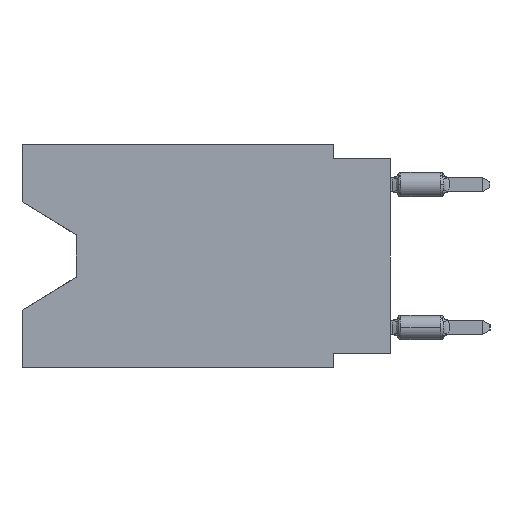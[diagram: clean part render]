
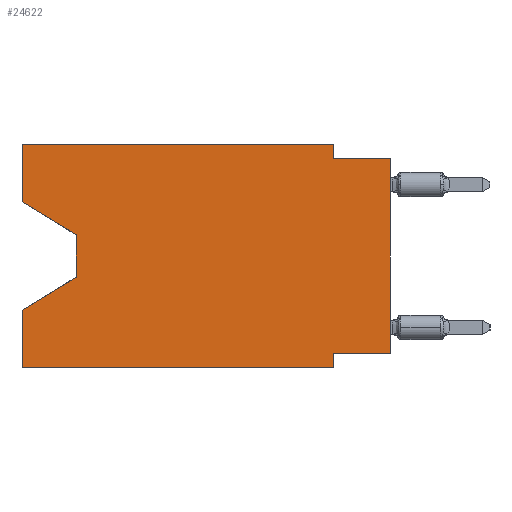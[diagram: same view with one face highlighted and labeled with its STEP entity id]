
A CAD part, left-side view. The second image highlights one B-rep face of the part: STEP entity #24622.
In plain terms, the highlighted planar face has unit normal (-1, 0, 0).
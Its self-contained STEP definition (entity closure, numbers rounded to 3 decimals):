
#47 = LINE ( 'NONE', #8810, #2737 ) ;
#103 = ORIENTED_EDGE ( 'NONE', *, *, #1691, .T. ) ;
#515 = ORIENTED_EDGE ( 'NONE', *, *, #9716, .T. ) ;
#597 = DIRECTION ( 'NONE',  ( 0., -1., 0. ) ) ;
#828 = VECTOR ( 'NONE', #20062, 1000. ) ;
#946 = VECTOR ( 'NONE', #24637, 1000. ) ;
#955 = VECTOR ( 'NONE', #1901, 1000. ) ;
#1691 = EDGE_CURVE ( 'NONE', #12206, #12368, #4442, .T. ) ;
#1764 = DIRECTION ( 'NONE',  ( 0., -1., 0. ) ) ;
#1812 = ORIENTED_EDGE ( 'NONE', *, *, #13598, .F. ) ;
#1901 = DIRECTION ( 'NONE',  ( 0., 0., 1. ) ) ;
#2100 = DIRECTION ( 'NONE',  ( 0., 0., -1. ) ) ;
#2536 = CARTESIAN_POINT ( 'NONE',  ( 0., 13.97, -4.013 ) ) ;
#2659 = CARTESIAN_POINT ( 'NONE',  ( 0., 0., -0.635 ) ) ;
#2737 = VECTOR ( 'NONE', #17561, 1000. ) ;
#2953 = DIRECTION ( 'NONE',  ( 0., 0., 1. ) ) ;
#3055 = VECTOR ( 'NONE', #597, 1000. ) ;
#3444 = VERTEX_POINT ( 'NONE', #13907 ) ;
#3875 = DIRECTION ( 'NONE',  ( 0., -1., 0. ) ) ;
#4442 = LINE ( 'NONE', #6744, #22879 ) ;
#4982 = ORIENTED_EDGE ( 'NONE', *, *, #12960, .F. ) ;
#4999 = CARTESIAN_POINT ( 'NONE',  ( 0., 2.54, -9.906 ) ) ;
#5498 = VERTEX_POINT ( 'NONE', #5629 ) ;
#5627 = CARTESIAN_POINT ( 'NONE',  ( 0., 2.54, -9.906 ) ) ;
#5629 = CARTESIAN_POINT ( 'NONE',  ( 0., 16.383, -7.36 ) ) ;
#5765 = EDGE_CURVE ( 'NONE', #12368, #5498, #17617, .T. ) ;
#6308 = VECTOR ( 'NONE', #7098, 1000. ) ;
#6665 = LINE ( 'NONE', #26929, #946 ) ;
#6677 = CARTESIAN_POINT ( 'NONE',  ( 0., 0., -9.271 ) ) ;
#6744 = CARTESIAN_POINT ( 'NONE',  ( 0., 13.97, -4.013 ) ) ;
#7058 = CARTESIAN_POINT ( 'NONE',  ( 0., 16.383, -9.906 ) ) ;
#7090 = AXIS2_PLACEMENT_3D ( 'NONE', #14928, #23681, #10766 ) ;
#7098 = DIRECTION ( 'NONE',  ( 0., 1., 0. ) ) ;
#7792 = LINE ( 'NONE', #5627, #11280 ) ;
#8624 = EDGE_CURVE ( 'NONE', #17166, #3444, #6665, .T. ) ;
#8719 = CARTESIAN_POINT ( 'NONE',  ( 0., 13.97, -5.893 ) ) ;
#8810 = CARTESIAN_POINT ( 'NONE',  ( 0., 16.383, -2.546 ) ) ;
#9716 = EDGE_CURVE ( 'NONE', #23384, #27047, #22628, .T. ) ;
#9970 = VERTEX_POINT ( 'NONE', #25915 ) ;
#10042 = VERTEX_POINT ( 'NONE', #20410 ) ;
#10766 = DIRECTION ( 'NONE',  ( 0., 0., -1. ) ) ;
#11064 = VECTOR ( 'NONE', #2100, 1000. ) ;
#11280 = VECTOR ( 'NONE', #14399, 1000. ) ;
#11384 = CARTESIAN_POINT ( 'NONE',  ( 0., 16.383, -2.546 ) ) ;
#11503 = VERTEX_POINT ( 'NONE', #23024 ) ;
#11617 = EDGE_CURVE ( 'NONE', #10042, #5498, #12825, .T. ) ;
#12206 = VERTEX_POINT ( 'NONE', #2536 ) ;
#12368 = VERTEX_POINT ( 'NONE', #27376 ) ;
#12781 = PLANE ( 'NONE',  #7090 ) ;
#12825 = LINE ( 'NONE', #25882, #955 ) ;
#12960 = EDGE_CURVE ( 'NONE', #3444, #11503, #19133, .T. ) ;
#13528 = ORIENTED_EDGE ( 'NONE', *, *, #17537, .T. ) ;
#13598 = EDGE_CURVE ( 'NONE', #11503, #18250, #17049, .T. ) ;
#13907 = CARTESIAN_POINT ( 'NONE',  ( 0., 16.383, 0. ) ) ;
#14399 = DIRECTION ( 'NONE',  ( 0., 0., -1. ) ) ;
#14800 = LINE ( 'NONE', #26674, #27342 ) ;
#14928 = CARTESIAN_POINT ( 'NONE',  ( 0., 16.383, 0. ) ) ;
#14962 = ORIENTED_EDGE ( 'NONE', *, *, #18263, .F. ) ;
#15528 = DIRECTION ( 'NONE',  ( 0., 0., -1. ) ) ;
#15753 = CARTESIAN_POINT ( 'NONE',  ( 0., 0., 0. ) ) ;
#16247 = EDGE_CURVE ( 'NONE', #18250, #27047, #14800, .T. ) ;
#17049 = LINE ( 'NONE', #21775, #11064 ) ;
#17166 = VERTEX_POINT ( 'NONE', #11384 ) ;
#17537 = EDGE_CURVE ( 'NONE', #10042, #28326, #22283, .T. ) ;
#17547 = CARTESIAN_POINT ( 'NONE',  ( 0., 16.383, 0. ) ) ;
#17561 = DIRECTION ( 'NONE',  ( 0., -0.855, -0.519 ) ) ;
#17617 = LINE ( 'NONE', #8719, #828 ) ;
#17756 = ORIENTED_EDGE ( 'NONE', *, *, #5765, .T. ) ;
#18024 = LINE ( 'NONE', #26782, #6308 ) ;
#18250 = VERTEX_POINT ( 'NONE', #24487 ) ;
#18263 = EDGE_CURVE ( 'NONE', #23384, #9970, #18024, .T. ) ;
#18760 = ORIENTED_EDGE ( 'NONE', *, *, #22827, .F. ) ;
#19133 = LINE ( 'NONE', #17547, #27996 ) ;
#19986 = ORIENTED_EDGE ( 'NONE', *, *, #8624, .F. ) ;
#20062 = DIRECTION ( 'NONE',  ( 0., 0.855, -0.519 ) ) ;
#20410 = CARTESIAN_POINT ( 'NONE',  ( 0., 16.383, -9.906 ) ) ;
#21775 = CARTESIAN_POINT ( 'NONE',  ( 0., 2.54, 0. ) ) ;
#22283 = LINE ( 'NONE', #7058, #3055 ) ;
#22628 = LINE ( 'NONE', #15753, #28312 ) ;
#22827 = EDGE_CURVE ( 'NONE', #9970, #28326, #7792, .T. ) ;
#22879 = VECTOR ( 'NONE', #15528, 1000. ) ;
#23024 = CARTESIAN_POINT ( 'NONE',  ( 0., 2.54, 0. ) ) ;
#23295 = ORIENTED_EDGE ( 'NONE', *, *, #16247, .F. ) ;
#23384 = VERTEX_POINT ( 'NONE', #6677 ) ;
#23681 = DIRECTION ( 'NONE',  ( 1., 0., 0. ) ) ;
#24487 = CARTESIAN_POINT ( 'NONE',  ( 0., 2.54, -0.635 ) ) ;
#24622 = ADVANCED_FACE ( 'NONE', ( #27715 ), #12781, .F. ) ;
#24637 = DIRECTION ( 'NONE',  ( 0., 0., 1. ) ) ;
#25882 = CARTESIAN_POINT ( 'NONE',  ( 0., 16.383, 0. ) ) ;
#25885 = ORIENTED_EDGE ( 'NONE', *, *, #11617, .F. ) ;
#25915 = CARTESIAN_POINT ( 'NONE',  ( 0., 2.54, -9.271 ) ) ;
#26433 = EDGE_LOOP ( 'NONE', ( #27167, #103, #17756, #25885, #13528, #18760, #14962, #515, #23295, #1812, #4982, #19986 ) ) ;
#26674 = CARTESIAN_POINT ( 'NONE',  ( 0., 0., -0.635 ) ) ;
#26782 = CARTESIAN_POINT ( 'NONE',  ( 0., 0., -9.271 ) ) ;
#26929 = CARTESIAN_POINT ( 'NONE',  ( 0., 16.383, 0. ) ) ;
#27047 = VERTEX_POINT ( 'NONE', #2659 ) ;
#27167 = ORIENTED_EDGE ( 'NONE', *, *, #27578, .T. ) ;
#27342 = VECTOR ( 'NONE', #3875, 1000. ) ;
#27376 = CARTESIAN_POINT ( 'NONE',  ( 0., 13.97, -5.893 ) ) ;
#27578 = EDGE_CURVE ( 'NONE', #17166, #12206, #47, .T. ) ;
#27715 = FACE_OUTER_BOUND ( 'NONE', #26433, .T. ) ;
#27996 = VECTOR ( 'NONE', #1764, 1000. ) ;
#28312 = VECTOR ( 'NONE', #2953, 1000. ) ;
#28326 = VERTEX_POINT ( 'NONE', #4999 ) ;
